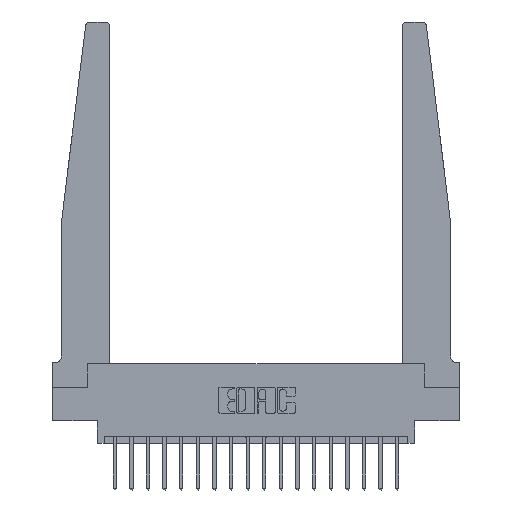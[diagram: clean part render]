
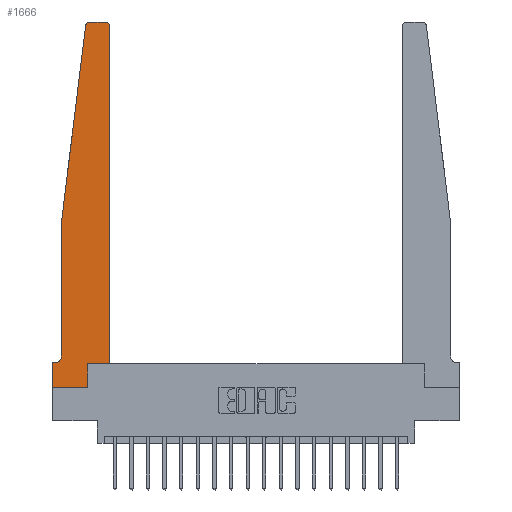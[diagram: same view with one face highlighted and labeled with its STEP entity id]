
A CAD part, top view. The second image highlights one B-rep face of the part: STEP entity #1666.
In plain terms, the highlighted planar face has unit normal (0, 0, 1).
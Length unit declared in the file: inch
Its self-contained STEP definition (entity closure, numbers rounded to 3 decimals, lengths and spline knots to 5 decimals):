
#17 = EDGE_CURVE ( 'NONE', #14143, #7224, #3948, .T. ) ;
#71 = DIRECTION ( 'NONE',  ( 0., 0., 1. ) ) ;
#702 = CARTESIAN_POINT ( 'NONE',  ( 0.395, 2.72, 0.37 ) ) ;
#724 = ORIENTED_EDGE ( 'NONE', *, *, #10019, .T. ) ;
#1645 = LINE ( 'NONE', #7933, #18509 ) ;
#1666 = ADVANCED_FACE ( 'NONE', ( #18692 ), #10900, .T. ) ;
#1780 = VECTOR ( 'NONE', #14794, 39.37008 ) ;
#2018 = CARTESIAN_POINT ( 'NONE',  ( 0.425, 2.72, 0.37 ) ) ;
#2224 = CARTESIAN_POINT ( 'NONE',  ( 0.2605, 0.18, 0.37 ) ) ;
#2344 = DIRECTION ( 'NONE',  ( 0., 0., 1. ) ) ;
#2559 = VERTEX_POINT ( 'NONE', #6326 ) ;
#2800 = VECTOR ( 'NONE', #16968, 39.37008 ) ;
#3003 = DIRECTION ( 'NONE',  ( -1., 0., 0. ) ) ;
#3058 = DIRECTION ( 'NONE',  ( 1., 0., 0. ) ) ;
#3356 = VECTOR ( 'NONE', #8722, 39.37008 ) ;
#3513 = CARTESIAN_POINT ( 'NONE',  ( 0.065, 1.25, 0.37 ) ) ;
#3633 = VERTEX_POINT ( 'NONE', #10740 ) ;
#3668 = EDGE_LOOP ( 'NONE', ( #724, #10852, #18573, #7620, #17836, #7753, #6343, #11609, #5506, #16093, #15431, #14017 ) ) ;
#3879 = VERTEX_POINT ( 'NONE', #12176 ) ;
#3948 = LINE ( 'NONE', #15050, #16312 ) ;
#4535 = LINE ( 'NONE', #6078, #2800 ) ;
#4649 = VERTEX_POINT ( 'NONE', #11738 ) ;
#5017 = VERTEX_POINT ( 'NONE', #2018 ) ;
#5403 = EDGE_CURVE ( 'NONE', #6153, #3633, #8820, .T. ) ;
#5506 = ORIENTED_EDGE ( 'NONE', *, *, #11704, .T. ) ;
#5724 = CARTESIAN_POINT ( 'NONE',  ( 0.2605, 0., 0.37 ) ) ;
#5757 = EDGE_CURVE ( 'NONE', #7224, #18562, #1645, .T. ) ;
#6014 = AXIS2_PLACEMENT_3D ( 'NONE', #12442, #71, #3058 ) ;
#6078 = CARTESIAN_POINT ( 'NONE',  ( 0.425, 0.18, 0.37 ) ) ;
#6103 = LINE ( 'NONE', #10937, #6837 ) ;
#6153 = VERTEX_POINT ( 'NONE', #8000 ) ;
#6326 = CARTESIAN_POINT ( 'NONE',  ( 0.065, 1.25, 0.37 ) ) ;
#6343 = ORIENTED_EDGE ( 'NONE', *, *, #17, .T. ) ;
#6465 = VERTEX_POINT ( 'NONE', #18170 ) ;
#6565 = EDGE_CURVE ( 'NONE', #2559, #4649, #10659, .T. ) ;
#6837 = VECTOR ( 'NONE', #3003, 39.37008 ) ;
#7101 = CARTESIAN_POINT ( 'NONE',  ( 0., 0.1875, 0.37 ) ) ;
#7176 = LINE ( 'NONE', #16745, #3356 ) ;
#7224 = VERTEX_POINT ( 'NONE', #18213 ) ;
#7620 = ORIENTED_EDGE ( 'NONE', *, *, #6565, .T. ) ;
#7753 = ORIENTED_EDGE ( 'NONE', *, *, #10687, .T. ) ;
#7933 = CARTESIAN_POINT ( 'NONE',  ( 0., 0., 0.37 ) ) ;
#8000 = CARTESIAN_POINT ( 'NONE',  ( 0.27653, 2.75, 0.37 ) ) ;
#8639 = DIRECTION ( 'NONE',  ( 1., 0., 0. ) ) ;
#8665 = CARTESIAN_POINT ( 'NONE',  ( 0.395, 2.75, 0.37 ) ) ;
#8671 = DIRECTION ( 'NONE',  ( 0., -1., 0. ) ) ;
#8698 = VERTEX_POINT ( 'NONE', #8665 ) ;
#8722 = DIRECTION ( 'NONE',  ( -1., 0., 0. ) ) ;
#8820 = CIRCLE ( 'NONE', #16376, 0.03 ) ;
#9119 = DIRECTION ( 'NONE',  ( 1., 0., 0. ) ) ;
#9778 = LINE ( 'NONE', #2224, #1780 ) ;
#10019 = EDGE_CURVE ( 'NONE', #8698, #6153, #6103, .T. ) ;
#10029 = CARTESIAN_POINT ( 'NONE',  ( 0.015, 0.1875, 0.37 ) ) ;
#10148 = EDGE_CURVE ( 'NONE', #3633, #2559, #14520, .T. ) ;
#10413 = CIRCLE ( 'NONE', #17957, 0.03 ) ;
#10499 = AXIS2_PLACEMENT_3D ( 'NONE', #20201, #16720, #10546 ) ;
#10546 = DIRECTION ( 'NONE',  ( -1., 0., 0. ) ) ;
#10552 = DIRECTION ( 'NONE',  ( 0., 0., 1. ) ) ;
#10659 = LINE ( 'NONE', #15391, #13336 ) ;
#10687 = EDGE_CURVE ( 'NONE', #20197, #14143, #7176, .T. ) ;
#10695 = DIRECTION ( 'NONE',  ( 0., 1., 0. ) ) ;
#10740 = CARTESIAN_POINT ( 'NONE',  ( 0.24675, 2.72367, 0.37 ) ) ;
#10817 = DIRECTION ( 'NONE',  ( 1., 0., 0. ) ) ;
#10852 = ORIENTED_EDGE ( 'NONE', *, *, #5403, .T. ) ;
#10900 = PLANE ( 'NONE',  #6014 ) ;
#10937 = CARTESIAN_POINT ( 'NONE',  ( 0.25, 2.75, 0.37 ) ) ;
#11109 = VECTOR ( 'NONE', #10695, 39.37008 ) ;
#11609 = ORIENTED_EDGE ( 'NONE', *, *, #5757, .T. ) ;
#11704 = EDGE_CURVE ( 'NONE', #18562, #6465, #9778, .T. ) ;
#11738 = CARTESIAN_POINT ( 'NONE',  ( 0.065, 0.2375, 0.37 ) ) ;
#12176 = CARTESIAN_POINT ( 'NONE',  ( 0.425, 0.18, 0.37 ) ) ;
#12442 = CARTESIAN_POINT ( 'NONE',  ( 0., 0.1875, 0.37 ) ) ;
#13336 = VECTOR ( 'NONE', #13951, 39.37008 ) ;
#13951 = DIRECTION ( 'NONE',  ( 0., -1., 0. ) ) ;
#13986 = CARTESIAN_POINT ( 'NONE',  ( 0.425, 0.18, 0.37 ) ) ;
#14017 = ORIENTED_EDGE ( 'NONE', *, *, #16445, .T. ) ;
#14143 = VERTEX_POINT ( 'NONE', #7101 ) ;
#14520 = LINE ( 'NONE', #3513, #19717 ) ;
#14794 = DIRECTION ( 'NONE',  ( 0., 1., 0. ) ) ;
#15050 = CARTESIAN_POINT ( 'NONE',  ( 0., 0., 0.37 ) ) ;
#15391 = CARTESIAN_POINT ( 'NONE',  ( 0.065, 1.25, 0.37 ) ) ;
#15431 = ORIENTED_EDGE ( 'NONE', *, *, #17795, .T. ) ;
#15435 = LINE ( 'NONE', #13986, #11109 ) ;
#15498 = CARTESIAN_POINT ( 'NONE',  ( 0.27653, 2.72, 0.37 ) ) ;
#15542 = EDGE_CURVE ( 'NONE', #6465, #3879, #4535, .T. ) ;
#16093 = ORIENTED_EDGE ( 'NONE', *, *, #15542, .T. ) ;
#16312 = VECTOR ( 'NONE', #8671, 39.37008 ) ;
#16376 = AXIS2_PLACEMENT_3D ( 'NONE', #15498, #10552, #9119 ) ;
#16445 = EDGE_CURVE ( 'NONE', #5017, #8698, #10413, .T. ) ;
#16720 = DIRECTION ( 'NONE',  ( 0., 0., -1. ) ) ;
#16745 = CARTESIAN_POINT ( 'NONE',  ( 0.065, 0.1875, 0.37 ) ) ;
#16968 = DIRECTION ( 'NONE',  ( 1., 0., 0. ) ) ;
#17703 = DIRECTION ( 'NONE',  ( -0.122, -0.992, 0. ) ) ;
#17795 = EDGE_CURVE ( 'NONE', #3879, #5017, #15435, .T. ) ;
#17836 = ORIENTED_EDGE ( 'NONE', *, *, #19925, .T. ) ;
#17957 = AXIS2_PLACEMENT_3D ( 'NONE', #702, #2344, #8639 ) ;
#18170 = CARTESIAN_POINT ( 'NONE',  ( 0.2605, 0.18, 0.37 ) ) ;
#18213 = CARTESIAN_POINT ( 'NONE',  ( 0., 0., 0.37 ) ) ;
#18509 = VECTOR ( 'NONE', #10817, 39.37008 ) ;
#18562 = VERTEX_POINT ( 'NONE', #5724 ) ;
#18573 = ORIENTED_EDGE ( 'NONE', *, *, #10148, .T. ) ;
#18692 = FACE_OUTER_BOUND ( 'NONE', #3668, .T. ) ;
#19046 = CIRCLE ( 'NONE', #10499, 0.05 ) ;
#19717 = VECTOR ( 'NONE', #17703, 39.37008 ) ;
#19925 = EDGE_CURVE ( 'NONE', #4649, #20197, #19046, .T. ) ;
#20197 = VERTEX_POINT ( 'NONE', #10029 ) ;
#20201 = CARTESIAN_POINT ( 'NONE',  ( 0.015, 0.2375, 0.37 ) ) ;
